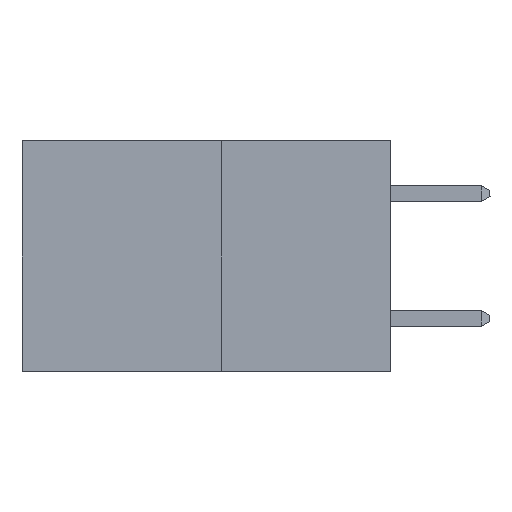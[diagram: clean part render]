
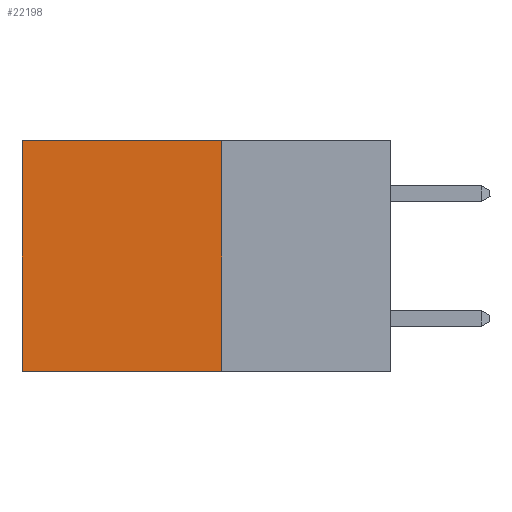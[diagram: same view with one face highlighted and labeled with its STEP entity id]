
A CAD part, left-side view. The second image highlights one B-rep face of the part: STEP entity #22198.
In plain terms, the highlighted planar face has unit normal (-1, 0, 0).
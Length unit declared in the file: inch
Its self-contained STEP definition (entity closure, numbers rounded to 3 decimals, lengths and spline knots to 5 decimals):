
#4 = PLANE ( 'NONE',  #8618 ) ;
#301 = EDGE_CURVE ( 'NONE', #25803, #20145, #10450, .T. ) ;
#411 = CARTESIAN_POINT ( 'NONE',  ( 0.277, 0.59, -0.37 ) ) ;
#2753 = DIRECTION ( 'NONE',  ( 0., 1., 0. ) ) ;
#2917 = CARTESIAN_POINT ( 'NONE',  ( 0.277, 0.27, 0. ) ) ;
#3172 = CARTESIAN_POINT ( 'NONE',  ( 0.277, 0.27, 0. ) ) ;
#4315 = DIRECTION ( 'NONE',  ( 1., 0., 0. ) ) ;
#5808 = VECTOR ( 'NONE', #7536, 39.37008 ) ;
#5821 = EDGE_CURVE ( 'NONE', #15111, #25803, #16815, .T. ) ;
#7536 = DIRECTION ( 'NONE',  ( 0., 0., -1. ) ) ;
#8303 = FACE_OUTER_BOUND ( 'NONE', #22640, .T. ) ;
#8381 = DIRECTION ( 'NONE',  ( 0., 0., -1. ) ) ;
#8618 = AXIS2_PLACEMENT_3D ( 'NONE', #16720, #4315, #18784 ) ;
#9498 = DIRECTION ( 'NONE',  ( 0., 1., 0. ) ) ;
#10450 = LINE ( 'NONE', #20439, #21398 ) ;
#11733 = ORIENTED_EDGE ( 'NONE', *, *, #14149, .T. ) ;
#11894 = ORIENTED_EDGE ( 'NONE', *, *, #19694, .T. ) ;
#12675 = VERTEX_POINT ( 'NONE', #17828 ) ;
#13957 = VECTOR ( 'NONE', #8381, 39.37008 ) ;
#14149 = EDGE_CURVE ( 'NONE', #12675, #20145, #18740, .T. ) ;
#14422 = ORIENTED_EDGE ( 'NONE', *, *, #5821, .F. ) ;
#15111 = VERTEX_POINT ( 'NONE', #2917 ) ;
#16720 = CARTESIAN_POINT ( 'NONE',  ( 0.277, 0.27, -0.37 ) ) ;
#16815 = LINE ( 'NONE', #24212, #5808 ) ;
#17828 = CARTESIAN_POINT ( 'NONE',  ( 0.277, 0.59, 0. ) ) ;
#18669 = CARTESIAN_POINT ( 'NONE',  ( 0.277, 0.59, -0.37 ) ) ;
#18740 = LINE ( 'NONE', #18669, #13957 ) ;
#18784 = DIRECTION ( 'NONE',  ( 0., 0., -1. ) ) ;
#19694 = EDGE_CURVE ( 'NONE', #15111, #12675, #19754, .T. ) ;
#19754 = LINE ( 'NONE', #3172, #24679 ) ;
#20145 = VERTEX_POINT ( 'NONE', #411 ) ;
#20439 = CARTESIAN_POINT ( 'NONE',  ( 0.277, 0.27, -0.37 ) ) ;
#20593 = ORIENTED_EDGE ( 'NONE', *, *, #301, .F. ) ;
#21398 = VECTOR ( 'NONE', #2753, 39.37008 ) ;
#21542 = CARTESIAN_POINT ( 'NONE',  ( 0.277, 0.27, -0.37 ) ) ;
#22198 = ADVANCED_FACE ( 'NONE', ( #8303 ), #4, .F. ) ;
#22640 = EDGE_LOOP ( 'NONE', ( #11733, #20593, #14422, #11894 ) ) ;
#24212 = CARTESIAN_POINT ( 'NONE',  ( 0.277, 0.27, -0.37 ) ) ;
#24679 = VECTOR ( 'NONE', #9498, 39.37008 ) ;
#25803 = VERTEX_POINT ( 'NONE', #21542 ) ;
